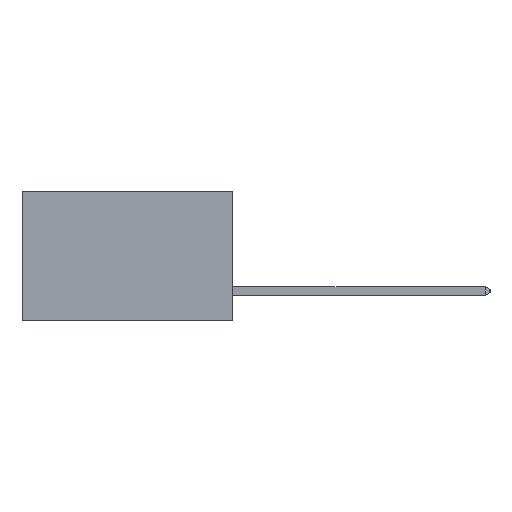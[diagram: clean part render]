
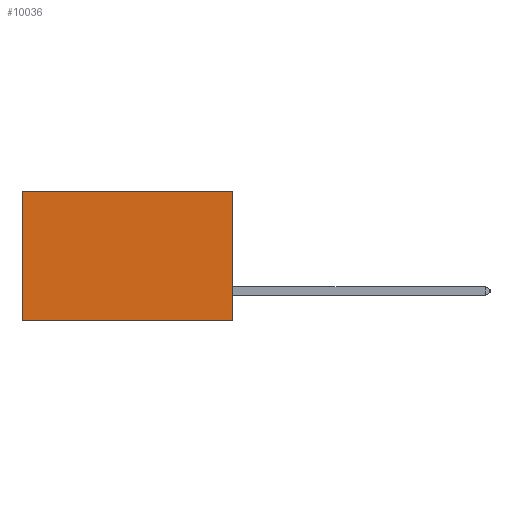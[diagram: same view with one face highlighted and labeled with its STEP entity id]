
A CAD part, left-side view. The second image highlights one B-rep face of the part: STEP entity #10036.
In plain terms, the highlighted planar face has unit normal (-1, 0, 0).
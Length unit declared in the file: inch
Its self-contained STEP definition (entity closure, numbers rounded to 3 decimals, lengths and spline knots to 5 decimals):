
#164 = ORIENTED_EDGE ( 'NONE', *, *, #6702, .T. ) ;
#2552 = CARTESIAN_POINT ( 'NONE',  ( 0.2875, 0., -0.37 ) ) ;
#2782 = DIRECTION ( 'NONE',  ( 0., 1., 0. ) ) ;
#5283 = LINE ( 'NONE', #26212, #13950 ) ;
#5646 = DIRECTION ( 'NONE',  ( 0., 0., -1. ) ) ;
#6044 = DIRECTION ( 'NONE',  ( 1., 0., 0. ) ) ;
#6311 = CARTESIAN_POINT ( 'NONE',  ( 0.2875, 0., 0. ) ) ;
#6612 = FACE_OUTER_BOUND ( 'NONE', #20596, .T. ) ;
#6702 = EDGE_CURVE ( 'NONE', #27251, #7593, #10574, .T. ) ;
#7593 = VERTEX_POINT ( 'NONE', #12525 ) ;
#8189 = VERTEX_POINT ( 'NONE', #8886 ) ;
#8886 = CARTESIAN_POINT ( 'NONE',  ( 0.2875, 0.6, -0.37 ) ) ;
#10036 = ADVANCED_FACE ( 'NONE', ( #6612 ), #16525, .F. ) ;
#10574 = LINE ( 'NONE', #15639, #23568 ) ;
#12525 = CARTESIAN_POINT ( 'NONE',  ( 0.2875, 0.6, 0. ) ) ;
#13298 = EDGE_CURVE ( 'NONE', #28855, #8189, #15415, .T. ) ;
#13950 = VECTOR ( 'NONE', #18353, 39.37008 ) ;
#15415 = LINE ( 'NONE', #2552, #21488 ) ;
#15639 = CARTESIAN_POINT ( 'NONE',  ( 0.2875, 0., 0. ) ) ;
#16357 = CARTESIAN_POINT ( 'NONE',  ( 0.2875, 0.6, 0. ) ) ;
#16525 = PLANE ( 'NONE',  #32248 ) ;
#18353 = DIRECTION ( 'NONE',  ( 0., 0., -1. ) ) ;
#18985 = DIRECTION ( 'NONE',  ( 0., 0., -1. ) ) ;
#19381 = ORIENTED_EDGE ( 'NONE', *, *, #23741, .F. ) ;
#19859 = VECTOR ( 'NONE', #18985, 39.37008 ) ;
#20596 = EDGE_LOOP ( 'NONE', ( #31738, #21531, #19381, #164 ) ) ;
#21488 = VECTOR ( 'NONE', #26123, 39.37008 ) ;
#21531 = ORIENTED_EDGE ( 'NONE', *, *, #13298, .F. ) ;
#22660 = EDGE_CURVE ( 'NONE', #7593, #8189, #31031, .T. ) ;
#23568 = VECTOR ( 'NONE', #2782, 39.37008 ) ;
#23741 = EDGE_CURVE ( 'NONE', #27251, #28855, #5283, .T. ) ;
#23897 = CARTESIAN_POINT ( 'NONE',  ( 0.2875, 0., 0. ) ) ;
#25948 = CARTESIAN_POINT ( 'NONE',  ( 0.2875, 0., -0.37 ) ) ;
#26123 = DIRECTION ( 'NONE',  ( 0., 1., 0. ) ) ;
#26212 = CARTESIAN_POINT ( 'NONE',  ( 0.2875, 0., 0. ) ) ;
#27251 = VERTEX_POINT ( 'NONE', #23897 ) ;
#28855 = VERTEX_POINT ( 'NONE', #25948 ) ;
#31031 = LINE ( 'NONE', #16357, #19859 ) ;
#31738 = ORIENTED_EDGE ( 'NONE', *, *, #22660, .T. ) ;
#32248 = AXIS2_PLACEMENT_3D ( 'NONE', #6311, #6044, #5646 ) ;
